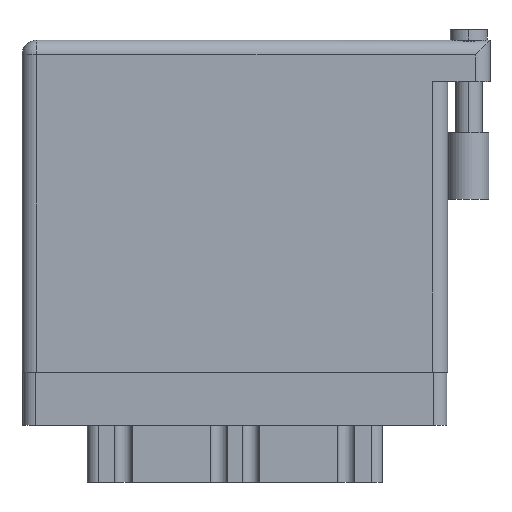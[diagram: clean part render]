
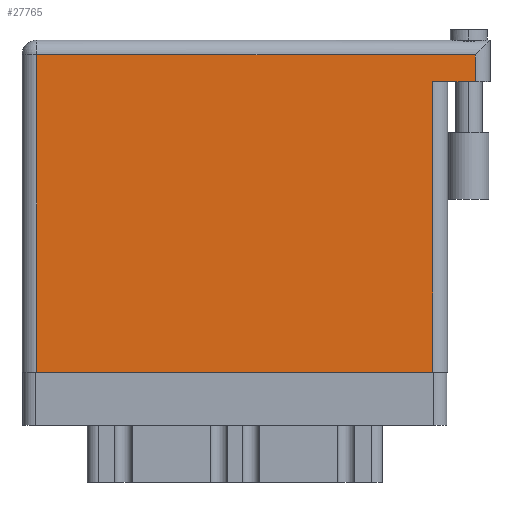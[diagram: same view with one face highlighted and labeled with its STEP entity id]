
A CAD part, front view. The second image highlights one B-rep face of the part: STEP entity #27765.
In plain terms, the highlighted face is planar.
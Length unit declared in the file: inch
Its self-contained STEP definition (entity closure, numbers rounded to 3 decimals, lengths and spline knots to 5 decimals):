
#78 = CARTESIAN_POINT ( 'NONE',  ( 2.138, 1.496, 0. ) ) ;
#998 = LINE ( 'NONE', #11962, #14008 ) ;
#1274 = LINE ( 'NONE', #12043, #16662 ) ;
#1560 = ORIENTED_EDGE ( 'NONE', *, *, #16245, .T. ) ;
#1946 = CARTESIAN_POINT ( 'NONE',  ( 1.938, 1.369, 0. ) ) ;
#2225 = EDGE_LOOP ( 'NONE', ( #1560, #23212, #20754, #27212, #3320, #29537 ) ) ;
#3320 = ORIENTED_EDGE ( 'NONE', *, *, #17711, .T. ) ;
#4332 = DIRECTION ( 'NONE',  ( 0., -1., 0. ) ) ;
#4726 = VERTEX_POINT ( 'NONE', #27126 ) ;
#4910 = EDGE_CURVE ( 'NONE', #20916, #28567, #15321, .T. ) ;
#5261 = CARTESIAN_POINT ( 'NONE',  ( 0., 1.496, 0. ) ) ;
#5676 = DIRECTION ( 'NONE',  ( 0., 1., 0. ) ) ;
#6250 = AXIS2_PLACEMENT_3D ( 'NONE', #10644, #15860, #23828 ) ;
#6542 = DIRECTION ( 'NONE',  ( -1., 0., 0. ) ) ;
#6885 = EDGE_CURVE ( 'NONE', #20916, #22649, #998, .T. ) ;
#6938 = LINE ( 'NONE', #17537, #27009 ) ;
#8301 = VERTEX_POINT ( 'NONE', #25203 ) ;
#10644 = CARTESIAN_POINT ( 'NONE',  ( 0., 1.566, 0. ) ) ;
#10899 = CARTESIAN_POINT ( 'NONE',  ( 1.938, 1.369, 0. ) ) ;
#11962 = CARTESIAN_POINT ( 'NONE',  ( 2.208, 1.369, 0. ) ) ;
#12043 = CARTESIAN_POINT ( 'NONE',  ( 0., 0., 0. ) ) ;
#12756 = LINE ( 'NONE', #5261, #21137 ) ;
#13238 = CARTESIAN_POINT ( 'NONE',  ( 2.138, 1.566, 0. ) ) ;
#13432 = CARTESIAN_POINT ( 'NONE',  ( 2.138, 1.369, 0. ) ) ;
#14008 = VECTOR ( 'NONE', #6542, 39.37008 ) ;
#15321 = LINE ( 'NONE', #13238, #16865 ) ;
#15350 = DIRECTION ( 'NONE',  ( -1., 0., 0. ) ) ;
#15860 = DIRECTION ( 'NONE',  ( 0., 0., -1. ) ) ;
#16245 = EDGE_CURVE ( 'NONE', #22870, #4726, #1274, .T. ) ;
#16662 = VECTOR ( 'NONE', #19671, 39.37008 ) ;
#16865 = VECTOR ( 'NONE', #26588, 39.37008 ) ;
#17537 = CARTESIAN_POINT ( 'NONE',  ( 0.07, 0., 0. ) ) ;
#17711 = EDGE_CURVE ( 'NONE', #28567, #8301, #12756, .T. ) ;
#18936 = CARTESIAN_POINT ( 'NONE',  ( 0.07, 0., 0. ) ) ;
#19671 = DIRECTION ( 'NONE',  ( 1., 0., 0. ) ) ;
#20754 = ORIENTED_EDGE ( 'NONE', *, *, #6885, .F. ) ;
#20916 = VERTEX_POINT ( 'NONE', #13432 ) ;
#21137 = VECTOR ( 'NONE', #15350, 39.37008 ) ;
#22649 = VERTEX_POINT ( 'NONE', #1946 ) ;
#22870 = VERTEX_POINT ( 'NONE', #18936 ) ;
#23212 = ORIENTED_EDGE ( 'NONE', *, *, #32629, .T. ) ;
#23828 = DIRECTION ( 'NONE',  ( -1., 0., 0. ) ) ;
#24103 = LINE ( 'NONE', #10899, #31526 ) ;
#24253 = EDGE_CURVE ( 'NONE', #8301, #22870, #6938, .T. ) ;
#25203 = CARTESIAN_POINT ( 'NONE',  ( 0.07, 1.496, 0. ) ) ;
#26588 = DIRECTION ( 'NONE',  ( 0., 1., 0. ) ) ;
#27009 = VECTOR ( 'NONE', #4332, 39.37008 ) ;
#27126 = CARTESIAN_POINT ( 'NONE',  ( 1.938, 0., 0. ) ) ;
#27212 = ORIENTED_EDGE ( 'NONE', *, *, #4910, .T. ) ;
#27765 = ADVANCED_FACE ( 'NONE', ( #31160 ), #31489, .F. ) ;
#28567 = VERTEX_POINT ( 'NONE', #78 ) ;
#29537 = ORIENTED_EDGE ( 'NONE', *, *, #24253, .T. ) ;
#31160 = FACE_OUTER_BOUND ( 'NONE', #2225, .T. ) ;
#31489 = PLANE ( 'NONE',  #6250 ) ;
#31526 = VECTOR ( 'NONE', #5676, 39.37008 ) ;
#32629 = EDGE_CURVE ( 'NONE', #4726, #22649, #24103, .T. ) ;
